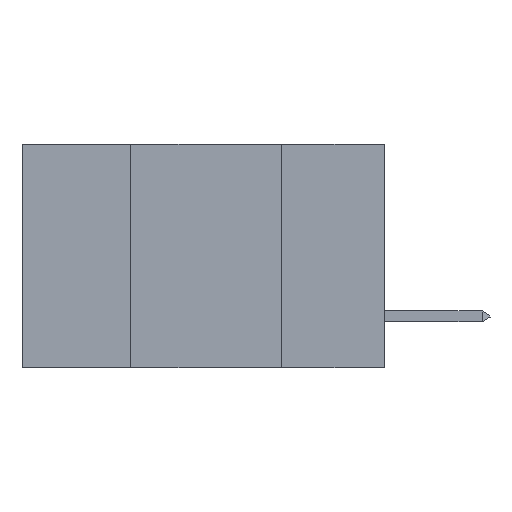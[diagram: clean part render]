
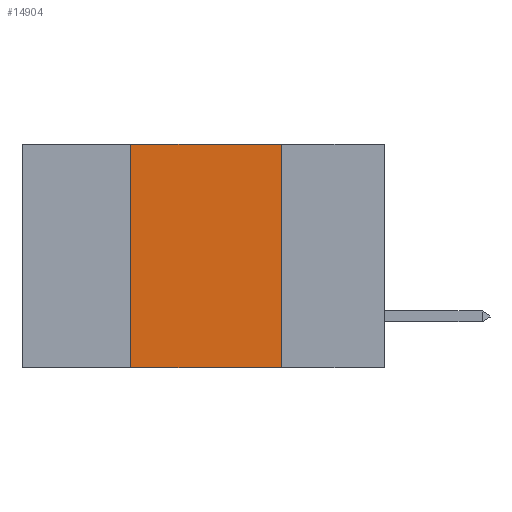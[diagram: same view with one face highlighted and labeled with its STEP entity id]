
A CAD part, left-side view. The second image highlights one B-rep face of the part: STEP entity #14904.
In plain terms, the highlighted planar face has unit normal (-1, 0, 0).
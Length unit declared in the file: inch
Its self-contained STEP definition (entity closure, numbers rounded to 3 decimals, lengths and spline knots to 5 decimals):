
#220 = CARTESIAN_POINT ( 'NONE',  ( 0., 0.42, -0.37 ) ) ;
#360 = CARTESIAN_POINT ( 'NONE',  ( 0., 0.42, 0. ) ) ;
#407 = DIRECTION ( 'NONE',  ( 0., 0., -1. ) ) ;
#1807 = VERTEX_POINT ( 'NONE', #19399 ) ;
#2320 = PLANE ( 'NONE',  #2411 ) ;
#2411 = AXIS2_PLACEMENT_3D ( 'NONE', #10560, #24770, #407 ) ;
#3006 = ORIENTED_EDGE ( 'NONE', *, *, #22631, .F. ) ;
#4115 = ORIENTED_EDGE ( 'NONE', *, *, #22211, .F. ) ;
#4592 = DIRECTION ( 'NONE',  ( 0., 0., 1. ) ) ;
#4598 = VECTOR ( 'NONE', #4592, 39.37008 ) ;
#6784 = VECTOR ( 'NONE', #19048, 39.37008 ) ;
#7017 = CARTESIAN_POINT ( 'NONE',  ( 0., 0.17, 0. ) ) ;
#7387 = EDGE_LOOP ( 'NONE', ( #3006, #4115, #21738, #22406 ) ) ;
#8541 = EDGE_CURVE ( 'NONE', #14927, #1807, #20468, .T. ) ;
#10560 = CARTESIAN_POINT ( 'NONE',  ( 0., 0.6, 0. ) ) ;
#11729 = VERTEX_POINT ( 'NONE', #22927 ) ;
#12023 = CARTESIAN_POINT ( 'NONE',  ( 0., 0.6, -0.37 ) ) ;
#14904 = ADVANCED_FACE ( 'NONE', ( #23290 ), #2320, .F. ) ;
#14927 = VERTEX_POINT ( 'NONE', #220 ) ;
#15714 = VERTEX_POINT ( 'NONE', #7017 ) ;
#15957 = EDGE_CURVE ( 'NONE', #14927, #11729, #23815, .T. ) ;
#16186 = DIRECTION ( 'NONE',  ( 0., -1., 0. ) ) ;
#16584 = LINE ( 'NONE', #18958, #6784 ) ;
#18958 = CARTESIAN_POINT ( 'NONE',  ( 0., 0.17, 0. ) ) ;
#19048 = DIRECTION ( 'NONE',  ( 0., 0., -1. ) ) ;
#19399 = CARTESIAN_POINT ( 'NONE',  ( 0., 0.42, 0. ) ) ;
#19465 = VECTOR ( 'NONE', #23729, 39.37008 ) ;
#19803 = CARTESIAN_POINT ( 'NONE',  ( 0., 0.6, 0. ) ) ;
#19982 = VECTOR ( 'NONE', #16186, 39.37008 ) ;
#20468 = LINE ( 'NONE', #360, #4598 ) ;
#21738 = ORIENTED_EDGE ( 'NONE', *, *, #8541, .F. ) ;
#22211 = EDGE_CURVE ( 'NONE', #1807, #15714, #24865, .T. ) ;
#22406 = ORIENTED_EDGE ( 'NONE', *, *, #15957, .T. ) ;
#22631 = EDGE_CURVE ( 'NONE', #15714, #11729, #16584, .T. ) ;
#22927 = CARTESIAN_POINT ( 'NONE',  ( 0., 0.17, -0.37 ) ) ;
#23290 = FACE_OUTER_BOUND ( 'NONE', #7387, .T. ) ;
#23729 = DIRECTION ( 'NONE',  ( 0., -1., 0. ) ) ;
#23815 = LINE ( 'NONE', #12023, #19982 ) ;
#24770 = DIRECTION ( 'NONE',  ( 1., 0., 0. ) ) ;
#24865 = LINE ( 'NONE', #19803, #19465 ) ;
